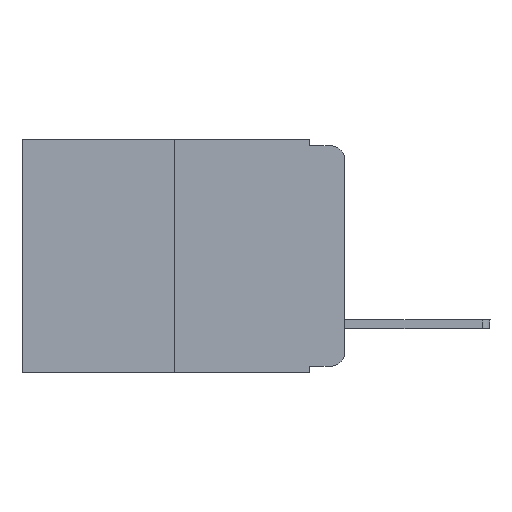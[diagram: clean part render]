
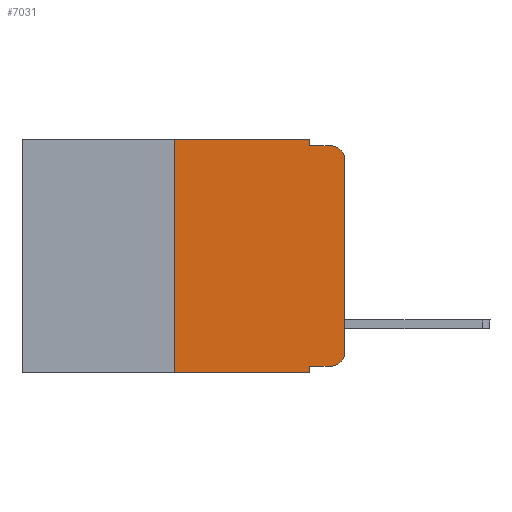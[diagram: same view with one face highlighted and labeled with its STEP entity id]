
A CAD part, left-side view. The second image highlights one B-rep face of the part: STEP entity #7031.
In plain terms, the highlighted planar face has unit normal (-1, 0, 0).
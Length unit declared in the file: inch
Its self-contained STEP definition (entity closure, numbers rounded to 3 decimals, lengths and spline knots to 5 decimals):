
#537 = VERTEX_POINT ( 'NONE', #10405 ) ;
#647 = CIRCLE ( 'NONE', #6384, 0.02 ) ;
#1055 = VERTEX_POINT ( 'NONE', #6691 ) ;
#1125 = EDGE_LOOP ( 'NONE', ( #16059, #6735, #8087, #1345, #13142, #16118, #2548, #4118, #6351, #2328 ) ) ;
#1345 = ORIENTED_EDGE ( 'NONE', *, *, #6985, .F. ) ;
#1347 = DIRECTION ( 'NONE',  ( 0., 0., -1. ) ) ;
#1749 = CIRCLE ( 'NONE', #6175, 0.02 ) ;
#1798 = CARTESIAN_POINT ( 'NONE',  ( 0., 0., 0. ) ) ;
#1858 = AXIS2_PLACEMENT_3D ( 'NONE', #2459, #11210, #12440 ) ;
#2011 = VERTEX_POINT ( 'NONE', #5987 ) ;
#2045 = CARTESIAN_POINT ( 'NONE',  ( 0., 0.051, -0.01 ) ) ;
#2165 = CARTESIAN_POINT ( 'NONE',  ( 0., 0.25, 0. ) ) ;
#2200 = VERTEX_POINT ( 'NONE', #16035 ) ;
#2328 = ORIENTED_EDGE ( 'NONE', *, *, #16020, .T. ) ;
#2459 = CARTESIAN_POINT ( 'NONE',  ( 0., 0.473, 0. ) ) ;
#2548 = ORIENTED_EDGE ( 'NONE', *, *, #5768, .T. ) ;
#2685 = CARTESIAN_POINT ( 'NONE',  ( 0., 0.473, -0.343 ) ) ;
#2882 = EDGE_CURVE ( 'NONE', #6537, #537, #11945, .T. ) ;
#2907 = DIRECTION ( 'NONE',  ( -1., 0., 0. ) ) ;
#2938 = VERTEX_POINT ( 'NONE', #13082 ) ;
#3005 = EDGE_CURVE ( 'NONE', #2938, #6243, #13402, .T. ) ;
#3034 = DIRECTION ( 'NONE',  ( 0., 0., -1. ) ) ;
#3262 = EDGE_CURVE ( 'NONE', #2011, #1055, #6908, .T. ) ;
#3272 = LINE ( 'NONE', #11777, #15520 ) ;
#3309 = DIRECTION ( 'NONE',  ( 0., 0., 1. ) ) ;
#3446 = DIRECTION ( 'NONE',  ( 0., 0., -1. ) ) ;
#3481 = CARTESIAN_POINT ( 'NONE',  ( 0., 0.051, 0. ) ) ;
#3586 = DIRECTION ( 'NONE',  ( 0., -1., 0. ) ) ;
#4118 = ORIENTED_EDGE ( 'NONE', *, *, #13414, .F. ) ;
#4170 = CARTESIAN_POINT ( 'NONE',  ( 0., 0., -0.03 ) ) ;
#4644 = EDGE_CURVE ( 'NONE', #1055, #12297, #10532, .T. ) ;
#5048 = VECTOR ( 'NONE', #8468, 39.37008 ) ;
#5324 = VERTEX_POINT ( 'NONE', #4170 ) ;
#5462 = DIRECTION ( 'NONE',  ( 0., -1., 0. ) ) ;
#5768 = EDGE_CURVE ( 'NONE', #2011, #5850, #7595, .T. ) ;
#5850 = VERTEX_POINT ( 'NONE', #6683 ) ;
#5987 = CARTESIAN_POINT ( 'NONE',  ( 0., 0.25, -0.343 ) ) ;
#6175 = AXIS2_PLACEMENT_3D ( 'NONE', #11439, #10227, #15351 ) ;
#6243 = VERTEX_POINT ( 'NONE', #11333 ) ;
#6351 = ORIENTED_EDGE ( 'NONE', *, *, #3005, .T. ) ;
#6384 = AXIS2_PLACEMENT_3D ( 'NONE', #15163, #2907, #1347 ) ;
#6537 = VERTEX_POINT ( 'NONE', #14677 ) ;
#6683 = CARTESIAN_POINT ( 'NONE',  ( 0., 0.051, -0.343 ) ) ;
#6691 = CARTESIAN_POINT ( 'NONE',  ( 0., 0.25, 0. ) ) ;
#6735 = ORIENTED_EDGE ( 'NONE', *, *, #12435, .T. ) ;
#6908 = LINE ( 'NONE', #2165, #10980 ) ;
#6985 = EDGE_CURVE ( 'NONE', #12297, #6537, #15859, .T. ) ;
#7031 = ADVANCED_FACE ( 'NONE', ( #14887 ), #12514, .F. ) ;
#7157 = EDGE_CURVE ( 'NONE', #2200, #5324, #9076, .T. ) ;
#7595 = LINE ( 'NONE', #2685, #13573 ) ;
#8087 = ORIENTED_EDGE ( 'NONE', *, *, #2882, .F. ) ;
#8090 = DIRECTION ( 'NONE',  ( 0., -1., 0. ) ) ;
#8468 = DIRECTION ( 'NONE',  ( 0., -1., 0. ) ) ;
#8911 = VECTOR ( 'NONE', #12919, 39.37008 ) ;
#9076 = LINE ( 'NONE', #1798, #8911 ) ;
#10085 = VECTOR ( 'NONE', #3586, 39.37008 ) ;
#10227 = DIRECTION ( 'NONE',  ( -1., 0., 0. ) ) ;
#10405 = CARTESIAN_POINT ( 'NONE',  ( 0., 0.02, -0.01 ) ) ;
#10532 = LINE ( 'NONE', #13386, #5048 ) ;
#10837 = VECTOR ( 'NONE', #8090, 39.37008 ) ;
#10893 = CARTESIAN_POINT ( 'NONE',  ( 0., 0.051, 0. ) ) ;
#10980 = VECTOR ( 'NONE', #3309, 39.37008 ) ;
#11210 = DIRECTION ( 'NONE',  ( 1., 0., 0. ) ) ;
#11333 = CARTESIAN_POINT ( 'NONE',  ( 0., 0.02, -0.333 ) ) ;
#11439 = CARTESIAN_POINT ( 'NONE',  ( 0., 0.02, -0.313 ) ) ;
#11777 = CARTESIAN_POINT ( 'NONE',  ( 0., 0.051, 0. ) ) ;
#11945 = LINE ( 'NONE', #2045, #10837 ) ;
#12297 = VERTEX_POINT ( 'NONE', #3481 ) ;
#12435 = EDGE_CURVE ( 'NONE', #5324, #537, #647, .T. ) ;
#12440 = DIRECTION ( 'NONE',  ( 0., 0., -1. ) ) ;
#12514 = PLANE ( 'NONE',  #1858 ) ;
#12919 = DIRECTION ( 'NONE',  ( 0., 0., 1. ) ) ;
#13082 = CARTESIAN_POINT ( 'NONE',  ( 0., 0.051, -0.333 ) ) ;
#13142 = ORIENTED_EDGE ( 'NONE', *, *, #4644, .F. ) ;
#13386 = CARTESIAN_POINT ( 'NONE',  ( 0., 0.473, 0. ) ) ;
#13402 = LINE ( 'NONE', #14708, #10085 ) ;
#13414 = EDGE_CURVE ( 'NONE', #2938, #5850, #3272, .T. ) ;
#13573 = VECTOR ( 'NONE', #5462, 39.37008 ) ;
#14677 = CARTESIAN_POINT ( 'NONE',  ( 0., 0.051, -0.01 ) ) ;
#14708 = CARTESIAN_POINT ( 'NONE',  ( 0., 0.051, -0.333 ) ) ;
#14887 = FACE_OUTER_BOUND ( 'NONE', #1125, .T. ) ;
#15163 = CARTESIAN_POINT ( 'NONE',  ( 0., 0.02, -0.03 ) ) ;
#15351 = DIRECTION ( 'NONE',  ( 0., 0., -1. ) ) ;
#15418 = VECTOR ( 'NONE', #3446, 39.37008 ) ;
#15520 = VECTOR ( 'NONE', #3034, 39.37008 ) ;
#15859 = LINE ( 'NONE', #10893, #15418 ) ;
#16020 = EDGE_CURVE ( 'NONE', #6243, #2200, #1749, .T. ) ;
#16035 = CARTESIAN_POINT ( 'NONE',  ( 0., 0., -0.313 ) ) ;
#16059 = ORIENTED_EDGE ( 'NONE', *, *, #7157, .T. ) ;
#16118 = ORIENTED_EDGE ( 'NONE', *, *, #3262, .F. ) ;
